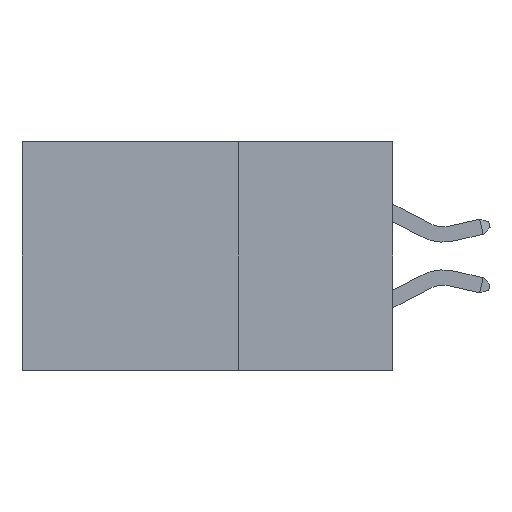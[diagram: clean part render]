
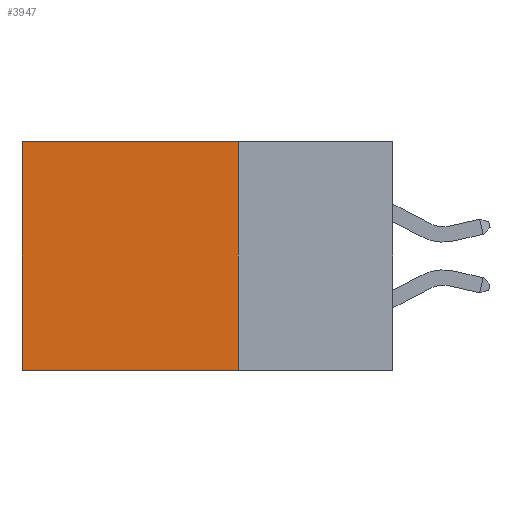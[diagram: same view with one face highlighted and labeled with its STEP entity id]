
A CAD part, left-side view. The second image highlights one B-rep face of the part: STEP entity #3947.
In plain terms, the highlighted planar face has unit normal (-1, 0, 0).
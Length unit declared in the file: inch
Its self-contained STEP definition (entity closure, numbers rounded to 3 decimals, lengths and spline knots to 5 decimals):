
#2616 = EDGE_LOOP ( 'NONE', ( #10065, #2644, #12767, #14065 ) ) ;
#2644 = ORIENTED_EDGE ( 'NONE', *, *, #3476, .F. ) ;
#2927 = FACE_OUTER_BOUND ( 'NONE', #2616, .T. ) ;
#3088 = VERTEX_POINT ( 'NONE', #12278 ) ;
#3476 = EDGE_CURVE ( 'NONE', #18042, #13598, #22800, .T. ) ;
#3947 = ADVANCED_FACE ( 'NONE', ( #2927 ), #23256, .F. ) ;
#4274 = CARTESIAN_POINT ( 'NONE',  ( 0.2875, 0.25, 0. ) ) ;
#4819 = EDGE_CURVE ( 'NONE', #14434, #3088, #22922, .T. ) ;
#5769 = VECTOR ( 'NONE', #21162, 39.37008 ) ;
#6085 = DIRECTION ( 'NONE',  ( 0., 0., -1. ) ) ;
#8022 = DIRECTION ( 'NONE',  ( 0., 1., 0. ) ) ;
#8238 = DIRECTION ( 'NONE',  ( 1., 0., 0. ) ) ;
#8991 = LINE ( 'NONE', #14586, #21759 ) ;
#9025 = CARTESIAN_POINT ( 'NONE',  ( 0.2875, 0.25, 0. ) ) ;
#9913 = LINE ( 'NONE', #23075, #12381 ) ;
#10065 = ORIENTED_EDGE ( 'NONE', *, *, #24077, .T. ) ;
#12278 = CARTESIAN_POINT ( 'NONE',  ( 0.2875, 0.6, 0. ) ) ;
#12381 = VECTOR ( 'NONE', #6085, 39.37008 ) ;
#12767 = ORIENTED_EDGE ( 'NONE', *, *, #14151, .F. ) ;
#13502 = CARTESIAN_POINT ( 'NONE',  ( 0.2875, 0.25, 0. ) ) ;
#13598 = VERTEX_POINT ( 'NONE', #19113 ) ;
#14065 = ORIENTED_EDGE ( 'NONE', *, *, #4819, .T. ) ;
#14124 = CARTESIAN_POINT ( 'NONE',  ( 0.2875, 0.25, -0.37 ) ) ;
#14151 = EDGE_CURVE ( 'NONE', #14434, #18042, #9913, .T. ) ;
#14434 = VERTEX_POINT ( 'NONE', #9025 ) ;
#14586 = CARTESIAN_POINT ( 'NONE',  ( 0.2875, 0.6, 0. ) ) ;
#17193 = CARTESIAN_POINT ( 'NONE',  ( 0.2875, 0.25, -0.37 ) ) ;
#18042 = VERTEX_POINT ( 'NONE', #14124 ) ;
#18827 = AXIS2_PLACEMENT_3D ( 'NONE', #4274, #8238, #23628 ) ;
#19113 = CARTESIAN_POINT ( 'NONE',  ( 0.2875, 0.6, -0.37 ) ) ;
#21162 = DIRECTION ( 'NONE',  ( 0., 1., 0. ) ) ;
#21759 = VECTOR ( 'NONE', #22155, 39.37008 ) ;
#22155 = DIRECTION ( 'NONE',  ( 0., 0., -1. ) ) ;
#22733 = VECTOR ( 'NONE', #8022, 39.37008 ) ;
#22800 = LINE ( 'NONE', #17193, #22733 ) ;
#22922 = LINE ( 'NONE', #13502, #5769 ) ;
#23075 = CARTESIAN_POINT ( 'NONE',  ( 0.2875, 0.25, 0. ) ) ;
#23256 = PLANE ( 'NONE',  #18827 ) ;
#23628 = DIRECTION ( 'NONE',  ( 0., 0., -1. ) ) ;
#24077 = EDGE_CURVE ( 'NONE', #3088, #13598, #8991, .T. ) ;
